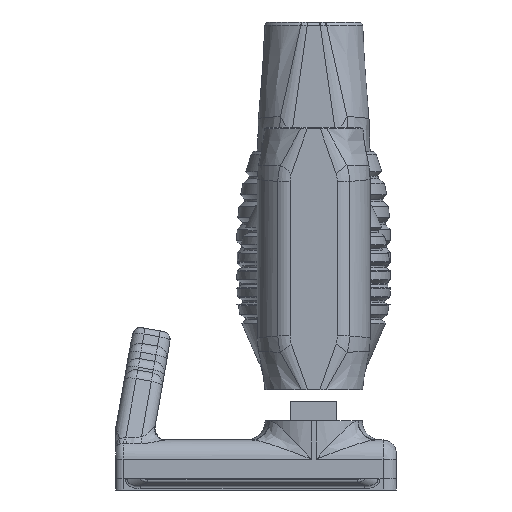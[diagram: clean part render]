
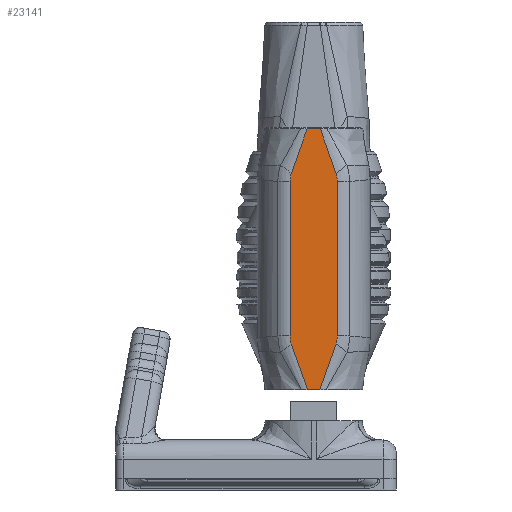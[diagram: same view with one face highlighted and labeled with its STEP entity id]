
A CAD part, left-side view. The second image highlights one B-rep face of the part: STEP entity #23141.
In plain terms, the highlighted planar face has unit normal (-1, 0, 0).
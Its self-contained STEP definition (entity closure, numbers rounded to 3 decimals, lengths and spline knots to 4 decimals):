
#1354=B_SPLINE_CURVE_WITH_KNOTS($,3,(#59570,#59571,#59572,#59573),
 .UNSPECIFIED.,.F.,.F.,(4,4),(-0.8391,0.0758),
 .UNSPECIFIED.);
#1355=B_SPLINE_CURVE_WITH_KNOTS($,3,(#59592,#59593,#59594,#59595),
 .UNSPECIFIED.,.F.,.F.,(4,4),(0.,0.1489),.UNSPECIFIED.);
#1358=B_SPLINE_CURVE_WITH_KNOTS($,3,(#59656,#59657,#59658,#59659),
 .UNSPECIFIED.,.F.,.F.,(4,4),(-0.0758,0.8391),
 .UNSPECIFIED.);
#1359=B_SPLINE_CURVE_WITH_KNOTS($,3,(#59679,#59680,#59681,#59682),
 .UNSPECIFIED.,.F.,.F.,(4,4),(0.,0.1489),.UNSPECIFIED.);
#1360=B_SPLINE_CURVE_WITH_KNOTS($,3,(#59699,#59700,#59701,#59702),
 .UNSPECIFIED.,.F.,.F.,(4,4),(0.,0.1489),.UNSPECIFIED.);
#1361=B_SPLINE_CURVE_WITH_KNOTS($,3,(#59704,#59705,#59706,#59707),
 .UNSPECIFIED.,.F.,.F.,(4,4),(-0.0449,0.8391),
 .UNSPECIFIED.);
#1362=B_SPLINE_CURVE_WITH_KNOTS($,3,(#59709,#59710,#59711,#59712),
 .UNSPECIFIED.,.F.,.F.,(4,4),(-0.1613,-0.1466),
 .UNSPECIFIED.);
#1363=B_SPLINE_CURVE_WITH_KNOTS($,3,(#59716,#59717,#59718,#59719),
 .UNSPECIFIED.,.F.,.F.,(4,4),(-0.0147,0.),.UNSPECIFIED.);
#1364=B_SPLINE_CURVE_WITH_KNOTS($,3,(#59721,#59722,#59723,#59724),
 .UNSPECIFIED.,.F.,.F.,(4,4),(-0.8391,0.0449),
 .UNSPECIFIED.);
#1365=B_SPLINE_CURVE_WITH_KNOTS($,3,(#59725,#59726,#59727,#59728),
 .UNSPECIFIED.,.F.,.F.,(4,4),(0.,0.1489),.UNSPECIFIED.);
#3173=LINE($,#59274,#4514);
#3174=LINE($,#59691,#4515);
#3176=LINE($,#59697,#4517);
#3177=LINE($,#59714,#4518);
#4514=VECTOR($,#30983,0.314);
#4515=VECTOR($,#31010,4.0172);
#4517=VECTOR($,#31016,4.0172);
#4518=VECTOR($,#31017,0.314);
#4951=PLANE($,#25364);
#6517=FACE_OUTER_BOUND($,#8113,.T.);
#8113=EDGE_LOOP($,(#21134,#21135,#21136,#21137,#21138,#21139,#21140,#21141,
#21142,#21143,#21144,#21145,#21146,#21147));
#11040=VERTEX_POINT($,#59265);
#11041=VERTEX_POINT($,#59273);
#11053=VERTEX_POINT($,#59568);
#11054=VERTEX_POINT($,#59590);
#11056=VERTEX_POINT($,#59655);
#11057=VERTEX_POINT($,#59677);
#11060=VERTEX_POINT($,#59690);
#11062=VERTEX_POINT($,#59696);
#11063=VERTEX_POINT($,#59698);
#11064=VERTEX_POINT($,#59703);
#11065=VERTEX_POINT($,#59708);
#11066=VERTEX_POINT($,#59713);
#11067=VERTEX_POINT($,#59715);
#11068=VERTEX_POINT($,#59720);
#14395=EDGE_CURVE($,#11040,#11041,#3173,.F.);
#14416=EDGE_CURVE($,#11053,#11040,#1354,.T.);
#14418=EDGE_CURVE($,#11054,#11053,#1355,.T.);
#14421=EDGE_CURVE($,#11041,#11056,#1358,.T.);
#14424=EDGE_CURVE($,#11056,#11057,#1359,.T.);
#14427=EDGE_CURVE($,#11057,#11060,#3174,.T.);
#14430=EDGE_CURVE($,#11062,#11054,#3176,.T.);
#14431=EDGE_CURVE($,#11063,#11062,#1360,.T.);
#14432=EDGE_CURVE($,#11064,#11063,#1361,.T.);
#14433=EDGE_CURVE($,#11065,#11064,#1362,.T.);
#14434=EDGE_CURVE($,#11066,#11065,#3177,.T.);
#14435=EDGE_CURVE($,#11067,#11066,#1363,.T.);
#14436=EDGE_CURVE($,#11068,#11067,#1364,.T.);
#14437=EDGE_CURVE($,#11060,#11068,#1365,.T.);
#21134=ORIENTED_EDGE($,*,*,#14430,.F.);
#21135=ORIENTED_EDGE($,*,*,#14431,.F.);
#21136=ORIENTED_EDGE($,*,*,#14432,.F.);
#21137=ORIENTED_EDGE($,*,*,#14433,.F.);
#21138=ORIENTED_EDGE($,*,*,#14434,.F.);
#21139=ORIENTED_EDGE($,*,*,#14435,.F.);
#21140=ORIENTED_EDGE($,*,*,#14436,.F.);
#21141=ORIENTED_EDGE($,*,*,#14437,.F.);
#21142=ORIENTED_EDGE($,*,*,#14427,.F.);
#21143=ORIENTED_EDGE($,*,*,#14424,.F.);
#21144=ORIENTED_EDGE($,*,*,#14421,.F.);
#21145=ORIENTED_EDGE($,*,*,#14395,.F.);
#21146=ORIENTED_EDGE($,*,*,#14416,.F.);
#21147=ORIENTED_EDGE($,*,*,#14418,.F.);
#23141=ADVANCED_FACE($,(#6517),#4951,.F.);
#25364=AXIS2_PLACEMENT_3D($,#59695,#31014,#31015);
#30983=DIRECTION($,(0.,-1.,0.));
#31010=DIRECTION($,(0.,0.,1.));
#31014=DIRECTION('center_axis',(1.,0.,0.));
#31015=DIRECTION('ref_axis',(0.,0.,-1.));
#31016=DIRECTION($,(0.,0.,-1.));
#31017=DIRECTION($,(0.,-1.,0.));
#59265=CARTESIAN_POINT('',(-12.8501,13.0321,2.3));
#59273=CARTESIAN_POINT('',(-12.8501,13.3461,2.3));
#59274=CARTESIAN_POINT($,(-12.8501,14.3535,2.3));
#59568=CARTESIAN_POINT('',(-12.8501,12.6083,3.493));
#59570=CARTESIAN_POINT('Ctrl Pts',(-12.8501,12.6083,3.493));
#59571=CARTESIAN_POINT('Ctrl Pts',(-12.8501,12.7458,3.0925));
#59572=CARTESIAN_POINT('Ctrl Pts',(-12.8501,12.8865,2.6943));
#59573=CARTESIAN_POINT('Ctrl Pts',(-12.8501,13.0321,2.3));
#59590=CARTESIAN_POINT('',(-12.8501,12.574,3.7042));
#59592=CARTESIAN_POINT('Ctrl Pts',(-12.8501,12.574,3.7042));
#59593=CARTESIAN_POINT('Ctrl Pts',(-12.8501,12.574,3.6312));
#59594=CARTESIAN_POINT('Ctrl Pts',(-12.8501,12.5859,3.5582));
#59595=CARTESIAN_POINT('Ctrl Pts',(-12.8501,12.6083,3.493));
#59655=CARTESIAN_POINT('',(-12.8501,13.7699,3.493));
#59656=CARTESIAN_POINT('Ctrl Pts',(-12.8501,13.3461,2.3));
#59657=CARTESIAN_POINT('Ctrl Pts',(-12.8501,13.4917,2.6943));
#59658=CARTESIAN_POINT('Ctrl Pts',(-12.8501,13.6324,3.0925));
#59659=CARTESIAN_POINT('Ctrl Pts',(-12.8501,13.7699,3.493));
#59677=CARTESIAN_POINT('',(-12.8501,13.8042,3.7042));
#59679=CARTESIAN_POINT('Ctrl Pts',(-12.8501,13.7699,3.493));
#59680=CARTESIAN_POINT('Ctrl Pts',(-12.8501,13.7923,3.5582));
#59681=CARTESIAN_POINT('Ctrl Pts',(-12.8501,13.8042,3.6312));
#59682=CARTESIAN_POINT('Ctrl Pts',(-12.8501,13.8042,3.7042));
#59690=CARTESIAN_POINT('',(-12.8501,13.8042,7.7214));
#59691=CARTESIAN_POINT($,(-12.8501,13.8042,7.9485));
#59695=CARTESIAN_POINT('Origin',(-12.8501,15.518,3.2187));
#59696=CARTESIAN_POINT('',(-12.8501,12.574,7.7214));
#59697=CARTESIAN_POINT($,(-12.8501,12.574,4.9485));
#59698=CARTESIAN_POINT('',(-12.8501,12.6083,7.9326));
#59699=CARTESIAN_POINT('Ctrl Pts',(-12.8501,12.6083,7.9326));
#59700=CARTESIAN_POINT('Ctrl Pts',(-12.8501,12.5859,7.8674));
#59701=CARTESIAN_POINT('Ctrl Pts',(-12.8501,12.574,7.7944));
#59702=CARTESIAN_POINT('Ctrl Pts',(-12.8501,12.574,7.7214));
#59703=CARTESIAN_POINT('',(-12.8501,13.0173,9.0856));
#59704=CARTESIAN_POINT('Ctrl Pts',(-12.8501,13.0173,9.0856));
#59705=CARTESIAN_POINT('Ctrl Pts',(-12.8501,12.877,8.7044));
#59706=CARTESIAN_POINT('Ctrl Pts',(-12.8501,12.7411,8.3196));
#59707=CARTESIAN_POINT('Ctrl Pts',(-12.8501,12.6083,7.9326));
#59708=CARTESIAN_POINT('',(-12.8501,13.0321,9.0856));
#59709=CARTESIAN_POINT('Ctrl Pts',(-12.8501,13.0321,9.0856));
#59710=CARTESIAN_POINT('Ctrl Pts',(-12.8501,13.0272,9.0856));
#59711=CARTESIAN_POINT('Ctrl Pts',(-12.8501,13.0223,9.0856));
#59712=CARTESIAN_POINT('Ctrl Pts',(-12.8501,13.0173,9.0856));
#59713=CARTESIAN_POINT('',(-12.8501,13.3461,9.0856));
#59714=CARTESIAN_POINT($,(-12.8501,14.3535,9.0856));
#59715=CARTESIAN_POINT('',(-12.8501,13.3608,9.0856));
#59716=CARTESIAN_POINT('Ctrl Pts',(-12.8501,13.3608,9.0856));
#59717=CARTESIAN_POINT('Ctrl Pts',(-12.8501,13.3559,9.0856));
#59718=CARTESIAN_POINT('Ctrl Pts',(-12.8501,13.351,9.0856));
#59719=CARTESIAN_POINT('Ctrl Pts',(-12.8501,13.3461,9.0856));
#59720=CARTESIAN_POINT('',(-12.8501,13.7699,7.9326));
#59721=CARTESIAN_POINT('Ctrl Pts',(-12.8501,13.7699,7.9326));
#59722=CARTESIAN_POINT('Ctrl Pts',(-12.8501,13.6371,8.3196));
#59723=CARTESIAN_POINT('Ctrl Pts',(-12.8501,13.5012,8.7044));
#59724=CARTESIAN_POINT('Ctrl Pts',(-12.8501,13.3608,9.0856));
#59725=CARTESIAN_POINT('Ctrl Pts',(-12.8501,13.8042,7.7214));
#59726=CARTESIAN_POINT('Ctrl Pts',(-12.8501,13.8042,7.7944));
#59727=CARTESIAN_POINT('Ctrl Pts',(-12.8501,13.7923,7.8674));
#59728=CARTESIAN_POINT('Ctrl Pts',(-12.8501,13.7699,7.9326));
